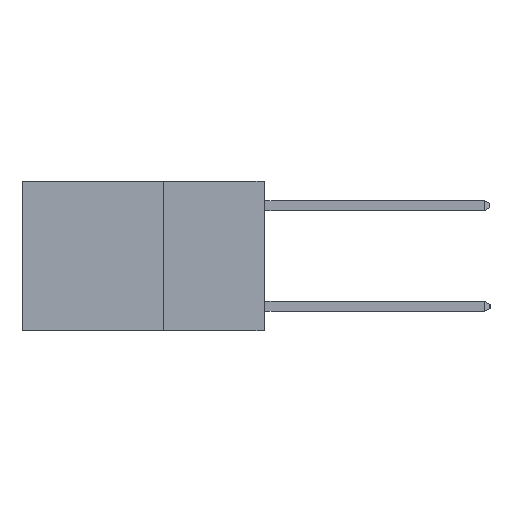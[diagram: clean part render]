
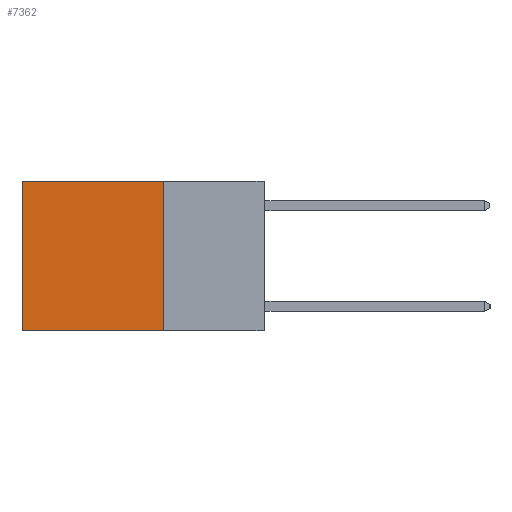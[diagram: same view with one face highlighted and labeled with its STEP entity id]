
A CAD part, left-side view. The second image highlights one B-rep face of the part: STEP entity #7362.
In plain terms, the highlighted planar face has unit normal (-1, 0, 0).
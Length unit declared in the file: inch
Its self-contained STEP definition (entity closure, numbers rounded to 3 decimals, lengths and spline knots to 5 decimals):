
#37 = ORIENTED_EDGE ( 'NONE', *, *, #4953, .T. ) ;
#749 = ORIENTED_EDGE ( 'NONE', *, *, #3888, .F. ) ;
#797 = VERTEX_POINT ( 'NONE', #6546 ) ;
#1050 = DIRECTION ( 'NONE',  ( 0., 0., -1. ) ) ;
#1176 = VECTOR ( 'NONE', #1050, 39.37008 ) ;
#1495 = CARTESIAN_POINT ( 'NONE',  ( 0.2625, 0.25, -0.37 ) ) ;
#1643 = DIRECTION ( 'NONE',  ( 0., 0., -1. ) ) ;
#1681 = EDGE_LOOP ( 'NONE', ( #9304, #6790, #749, #37 ) ) ;
#1796 = DIRECTION ( 'NONE',  ( 0., 0., -1. ) ) ;
#2341 = EDGE_CURVE ( 'NONE', #11624, #7509, #5371, .T. ) ;
#2350 = VECTOR ( 'NONE', #1643, 39.37008 ) ;
#3888 = EDGE_CURVE ( 'NONE', #797, #11624, #11695, .T. ) ;
#4039 = CARTESIAN_POINT ( 'NONE',  ( 0.2625, 0.25, 0. ) ) ;
#4052 = VERTEX_POINT ( 'NONE', #11771 ) ;
#4843 = FACE_OUTER_BOUND ( 'NONE', #1681, .T. ) ;
#4953 = EDGE_CURVE ( 'NONE', #797, #4052, #8484, .T. ) ;
#5371 = LINE ( 'NONE', #5488, #10184 ) ;
#5426 = EDGE_CURVE ( 'NONE', #4052, #7509, #10554, .T. ) ;
#5488 = CARTESIAN_POINT ( 'NONE',  ( 0.2625, 0.25, -0.37 ) ) ;
#5661 = CARTESIAN_POINT ( 'NONE',  ( 0.2625, 0.6, 0. ) ) ;
#5774 = VECTOR ( 'NONE', #7746, 39.37008 ) ;
#6370 = CARTESIAN_POINT ( 'NONE',  ( 0.2625, 0.25, 0. ) ) ;
#6546 = CARTESIAN_POINT ( 'NONE',  ( 0.2625, 0.25, 0. ) ) ;
#6790 = ORIENTED_EDGE ( 'NONE', *, *, #2341, .F. ) ;
#7144 = CARTESIAN_POINT ( 'NONE',  ( 0.2625, 0.25, 0. ) ) ;
#7301 = DIRECTION ( 'NONE',  ( 1., 0., 0. ) ) ;
#7362 = ADVANCED_FACE ( 'NONE', ( #4843 ), #11713, .F. ) ;
#7509 = VERTEX_POINT ( 'NONE', #8385 ) ;
#7746 = DIRECTION ( 'NONE',  ( 0., 1., 0. ) ) ;
#8385 = CARTESIAN_POINT ( 'NONE',  ( 0.2625, 0.6, -0.37 ) ) ;
#8484 = LINE ( 'NONE', #4039, #5774 ) ;
#9304 = ORIENTED_EDGE ( 'NONE', *, *, #5426, .T. ) ;
#9570 = AXIS2_PLACEMENT_3D ( 'NONE', #6370, #7301, #1796 ) ;
#10184 = VECTOR ( 'NONE', #11767, 39.37008 ) ;
#10554 = LINE ( 'NONE', #5661, #1176 ) ;
#11624 = VERTEX_POINT ( 'NONE', #1495 ) ;
#11695 = LINE ( 'NONE', #7144, #2350 ) ;
#11713 = PLANE ( 'NONE',  #9570 ) ;
#11767 = DIRECTION ( 'NONE',  ( 0., 1., 0. ) ) ;
#11771 = CARTESIAN_POINT ( 'NONE',  ( 0.2625, 0.6, 0. ) ) ;
